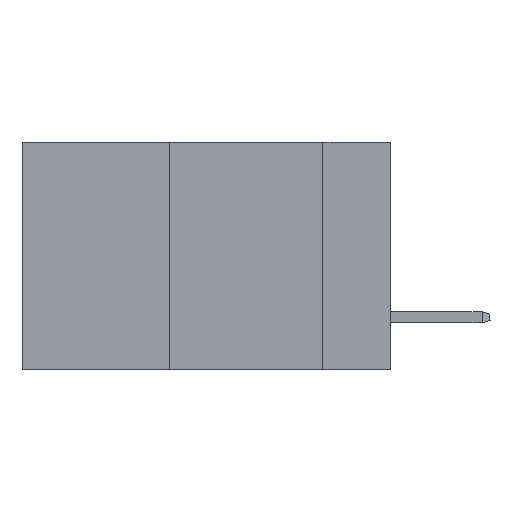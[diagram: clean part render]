
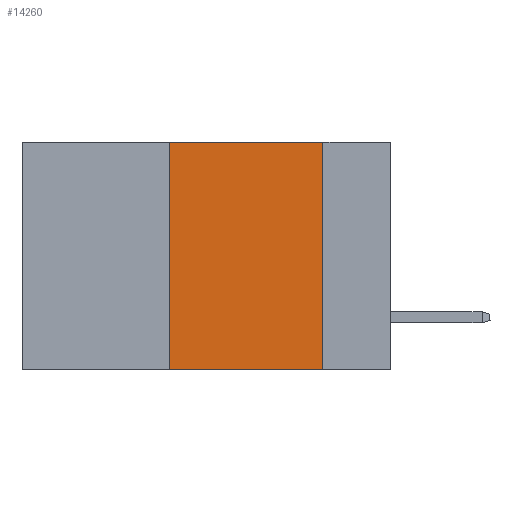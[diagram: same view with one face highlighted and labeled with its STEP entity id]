
A CAD part, left-side view. The second image highlights one B-rep face of the part: STEP entity #14260.
In plain terms, the highlighted planar face has unit normal (-1, 0, 0).
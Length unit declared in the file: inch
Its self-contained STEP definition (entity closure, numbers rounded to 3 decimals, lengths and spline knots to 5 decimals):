
#1437 = FACE_OUTER_BOUND ( 'NONE', #19125, .T. ) ;
#2000 = ORIENTED_EDGE ( 'NONE', *, *, #18061, .F. ) ;
#2919 = VERTEX_POINT ( 'NONE', #4504 ) ;
#3157 = ORIENTED_EDGE ( 'NONE', *, *, #19705, .F. ) ;
#3651 = CARTESIAN_POINT ( 'NONE',  ( 0., 0.11, 0. ) ) ;
#4126 = DIRECTION ( 'NONE',  ( 0., 0., 1. ) ) ;
#4504 = CARTESIAN_POINT ( 'NONE',  ( 0., 0.36, -0.37 ) ) ;
#6062 = VERTEX_POINT ( 'NONE', #34745 ) ;
#6236 = DIRECTION ( 'NONE',  ( 0., -1., 0. ) ) ;
#9280 = CARTESIAN_POINT ( 'NONE',  ( 0., 0.6, -0.37 ) ) ;
#11919 = ORIENTED_EDGE ( 'NONE', *, *, #29473, .F. ) ;
#13011 = LINE ( 'NONE', #40072, #23667 ) ;
#14260 = ADVANCED_FACE ( 'NONE', ( #1437 ), #24552, .F. ) ;
#15505 = VERTEX_POINT ( 'NONE', #31234 ) ;
#17202 = CARTESIAN_POINT ( 'NONE',  ( 0., 0.6, 0. ) ) ;
#18061 = EDGE_CURVE ( 'NONE', #23909, #6062, #24696, .T. ) ;
#19125 = EDGE_LOOP ( 'NONE', ( #2000, #3157, #11919, #24451 ) ) ;
#19611 = LINE ( 'NONE', #9280, #37595 ) ;
#19688 = VECTOR ( 'NONE', #42921, 39.37008 ) ;
#19705 = EDGE_CURVE ( 'NONE', #15505, #23909, #26975, .T. ) ;
#23667 = VECTOR ( 'NONE', #4126, 39.37008 ) ;
#23909 = VERTEX_POINT ( 'NONE', #39441 ) ;
#24451 = ORIENTED_EDGE ( 'NONE', *, *, #35669, .T. ) ;
#24552 = PLANE ( 'NONE',  #41439 ) ;
#24696 = LINE ( 'NONE', #3651, #19688 ) ;
#26975 = LINE ( 'NONE', #34853, #35436 ) ;
#29473 = EDGE_CURVE ( 'NONE', #2919, #15505, #13011, .T. ) ;
#31234 = CARTESIAN_POINT ( 'NONE',  ( 0., 0.36, 0. ) ) ;
#31967 = DIRECTION ( 'NONE',  ( 0., 0., -1. ) ) ;
#34745 = CARTESIAN_POINT ( 'NONE',  ( 0., 0.11, -0.37 ) ) ;
#34853 = CARTESIAN_POINT ( 'NONE',  ( 0., 0.6, 0. ) ) ;
#35154 = DIRECTION ( 'NONE',  ( 0., -1., 0. ) ) ;
#35436 = VECTOR ( 'NONE', #35154, 39.37008 ) ;
#35669 = EDGE_CURVE ( 'NONE', #2919, #6062, #19611, .T. ) ;
#37595 = VECTOR ( 'NONE', #6236, 39.37008 ) ;
#39441 = CARTESIAN_POINT ( 'NONE',  ( 0., 0.11, 0. ) ) ;
#40072 = CARTESIAN_POINT ( 'NONE',  ( 0., 0.36, 0. ) ) ;
#41439 = AXIS2_PLACEMENT_3D ( 'NONE', #17202, #42340, #31967 ) ;
#42340 = DIRECTION ( 'NONE',  ( 1., 0., 0. ) ) ;
#42921 = DIRECTION ( 'NONE',  ( 0., 0., -1. ) ) ;
